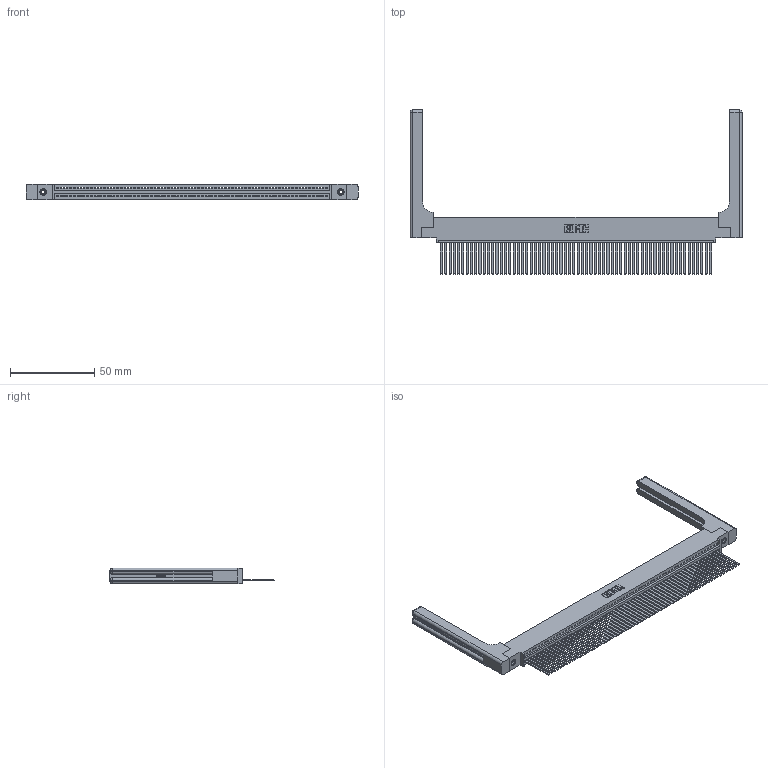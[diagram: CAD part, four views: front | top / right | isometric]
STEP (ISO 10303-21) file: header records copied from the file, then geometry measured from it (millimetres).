
FILE_DESCRIPTION (( 'STEP AP203' ), '1' );
FILE_NAME ('395-064-544-458.STEP', '2019-10-25T03:22:35', ( '' ), ( '' ), 'SwSTEP 2.0', 'SolidWorks 2016', '' );
FILE_SCHEMA (( 'CONFIG_CONTROL_DESIGN' ));
Length unit declared in the file: inch
Products named in the file (5): 345-250-001_345-250-001-102; 345 Part_0.110 Offset - 0.156 Dia-TH; 395-064-544-458; 345-220-058_345-220-058; 345-292-001_345-293-144
Assembly tree (69 placements, depth 2):
  395-064-544-458
    345 Part_0.110 Offset - 0.156 Dia-TH
    345-292-001_345-293-144  x64
    345-250-001_345-250-001-102  x2
    345-220-058_345-220-058  x2
Bounding box: 197.59 x 97.71 x 9.4 mm (x, y, z)
Volume: 28120 mm3; surface area: 33978.2 mm2
Topology: 69 solids, 69 shells, 3714 faces, 11131 edges, 7314 vertices
Faces by surface type: plane 2536, cylinder 1118, bspline 36, cone 12, sphere 8, torus 4
Entity records: 50336 total; most frequent: CARTESIAN_POINT 9689, ORIENTED_EDGE 8484, DIRECTION 7374, EDGE_CURVE 4242, VECTOR 3766, LINE 3766, VERTEX_POINT 2818, AXIS2_PLACEMENT_3D 1804
